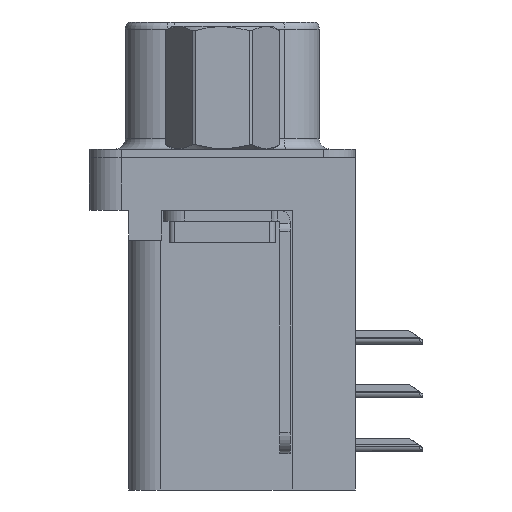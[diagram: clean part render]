
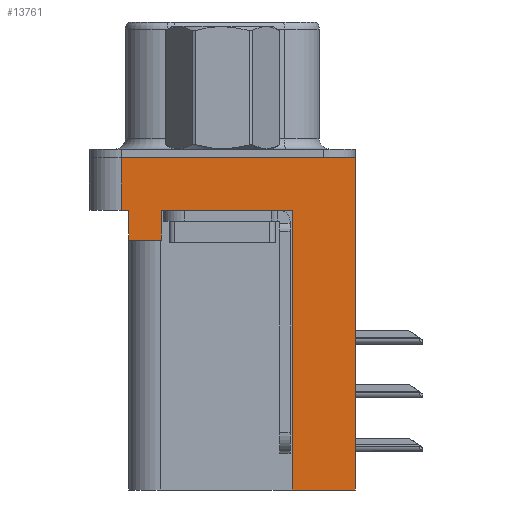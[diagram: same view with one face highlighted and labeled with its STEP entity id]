
A CAD part, left-side view. The second image highlights one B-rep face of the part: STEP entity #13761.
In plain terms, the highlighted planar face has unit normal (-1, 0, 0).
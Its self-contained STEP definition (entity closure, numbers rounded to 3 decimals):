
#424 = VERTEX_POINT ( 'NONE', #17950 ) ;
#439 = CARTESIAN_POINT ( 'NONE',  ( -2.91, 4.425, -3.9 ) ) ;
#512 = LINE ( 'NONE', #6853, #30821 ) ;
#1835 = EDGE_CURVE ( 'NONE', #17259, #18678, #512, .T. ) ;
#2288 = VECTOR ( 'NONE', #24441, 1000. ) ;
#3226 = CARTESIAN_POINT ( 'NONE',  ( -2.91, 4.425, -3.9 ) ) ;
#3287 = VERTEX_POINT ( 'NONE', #3580 ) ;
#3580 = CARTESIAN_POINT ( 'NONE',  ( -2.91, -3.295, -2.5 ) ) ;
#4330 = CARTESIAN_POINT ( 'NONE',  ( -2.91, -3.295, -15.7 ) ) ;
#4665 = ORIENTED_EDGE ( 'NONE', *, *, #38914, .T. ) ;
#4930 = CARTESIAN_POINT ( 'NONE',  ( -2.91, 4.775, -2.5 ) ) ;
#5229 = DIRECTION ( 'NONE',  ( 0., 0., 1. ) ) ;
#5302 = EDGE_CURVE ( 'NONE', #17259, #13470, #11109, .T. ) ;
#5963 = CARTESIAN_POINT ( 'NONE',  ( -2.91, 2.895, -2.5 ) ) ;
#6119 = ORIENTED_EDGE ( 'NONE', *, *, #8988, .F. ) ;
#6169 = DIRECTION ( 'NONE',  ( 0., 0., 1. ) ) ;
#6502 = DIRECTION ( 'NONE',  ( 0., 0., 1. ) ) ;
#6520 = CARTESIAN_POINT ( 'NONE',  ( -2.91, 4.775, 0. ) ) ;
#6759 = AXIS2_PLACEMENT_3D ( 'NONE', #12390, #24527, #6502 ) ;
#6853 = CARTESIAN_POINT ( 'NONE',  ( -2.91, 2.895, -3.9 ) ) ;
#7241 = EDGE_CURVE ( 'NONE', #424, #34237, #39481, .T. ) ;
#7870 = DIRECTION ( 'NONE',  ( 0., 0., 1. ) ) ;
#8988 = EDGE_CURVE ( 'NONE', #25546, #35656, #13294, .T. ) ;
#9423 = LINE ( 'NONE', #17387, #32931 ) ;
#9431 = ORIENTED_EDGE ( 'NONE', *, *, #9508, .F. ) ;
#9508 = EDGE_CURVE ( 'NONE', #424, #25546, #15098, .T. ) ;
#9706 = DIRECTION ( 'NONE',  ( 0., 0., 1. ) ) ;
#9744 = EDGE_CURVE ( 'NONE', #13470, #34237, #10437, .T. ) ;
#10287 = EDGE_CURVE ( 'NONE', #25316, #3287, #9423, .T. ) ;
#10437 = LINE ( 'NONE', #3226, #25574 ) ;
#10825 = EDGE_CURVE ( 'NONE', #34011, #25316, #37841, .T. ) ;
#11051 = EDGE_CURVE ( 'NONE', #34011, #35656, #38979, .T. ) ;
#11109 = LINE ( 'NONE', #439, #2288 ) ;
#11117 = ORIENTED_EDGE ( 'NONE', *, *, #5302, .F. ) ;
#11288 = ORIENTED_EDGE ( 'NONE', *, *, #11051, .T. ) ;
#12390 = CARTESIAN_POINT ( 'NONE',  ( -2.91, -6.275, -2.5 ) ) ;
#13294 = LINE ( 'NONE', #30433, #36029 ) ;
#13470 = VERTEX_POINT ( 'NONE', #31010 ) ;
#13516 = CARTESIAN_POINT ( 'NONE',  ( -2.91, 4.425, -2.5 ) ) ;
#13761 = ADVANCED_FACE ( 'NONE', ( #30510 ), #21433, .T. ) ;
#14116 = VECTOR ( 'NONE', #16298, 1000. ) ;
#15098 = LINE ( 'NONE', #4930, #30489 ) ;
#15733 = CARTESIAN_POINT ( 'NONE',  ( -2.91, -6.275, -2.5 ) ) ;
#16298 = DIRECTION ( 'NONE',  ( 0., 1., 0. ) ) ;
#16549 = LINE ( 'NONE', #24959, #23657 ) ;
#17077 = CARTESIAN_POINT ( 'NONE',  ( -2.91, -6.275, -2.5 ) ) ;
#17259 = VERTEX_POINT ( 'NONE', #36626 ) ;
#17279 = CARTESIAN_POINT ( 'NONE',  ( -2.91, -3.295, -15.7 ) ) ;
#17387 = CARTESIAN_POINT ( 'NONE',  ( -2.91, -3.295, -15.7 ) ) ;
#17950 = CARTESIAN_POINT ( 'NONE',  ( -2.91, 4.775, -2.5 ) ) ;
#18678 = VERTEX_POINT ( 'NONE', #5963 ) ;
#19077 = DIRECTION ( 'NONE',  ( 0., -1., 0. ) ) ;
#20397 = DIRECTION ( 'NONE',  ( 0., 0., 1. ) ) ;
#21433 = PLANE ( 'NONE',  #6759 ) ;
#23657 = VECTOR ( 'NONE', #19077, 1000. ) ;
#24296 = ORIENTED_EDGE ( 'NONE', *, *, #10825, .F. ) ;
#24441 = DIRECTION ( 'NONE',  ( 0., 1., 0. ) ) ;
#24527 = DIRECTION ( 'NONE',  ( -1., 0., 0. ) ) ;
#24959 = CARTESIAN_POINT ( 'NONE',  ( -2.91, -6.275, -2.5 ) ) ;
#25316 = VERTEX_POINT ( 'NONE', #17279 ) ;
#25546 = VERTEX_POINT ( 'NONE', #6520 ) ;
#25574 = VECTOR ( 'NONE', #6169, 1000. ) ;
#27241 = CARTESIAN_POINT ( 'NONE',  ( -2.91, -6.275, -15.7 ) ) ;
#28014 = ORIENTED_EDGE ( 'NONE', *, *, #1835, .T. ) ;
#30433 = CARTESIAN_POINT ( 'NONE',  ( -2.91, -6.275, 0. ) ) ;
#30489 = VECTOR ( 'NONE', #7870, 1000. ) ;
#30510 = FACE_OUTER_BOUND ( 'NONE', #39090, .T. ) ;
#30581 = VECTOR ( 'NONE', #5229, 1000. ) ;
#30821 = VECTOR ( 'NONE', #9706, 1000. ) ;
#31010 = CARTESIAN_POINT ( 'NONE',  ( -2.91, 4.425, -3.9 ) ) ;
#31056 = DIRECTION ( 'NONE',  ( 0., -1., 0. ) ) ;
#31685 = ORIENTED_EDGE ( 'NONE', *, *, #7241, .T. ) ;
#32931 = VECTOR ( 'NONE', #20397, 1000. ) ;
#33631 = DIRECTION ( 'NONE',  ( 0., -1., 0. ) ) ;
#34011 = VERTEX_POINT ( 'NONE', #27241 ) ;
#34237 = VERTEX_POINT ( 'NONE', #13516 ) ;
#35656 = VERTEX_POINT ( 'NONE', #36658 ) ;
#36029 = VECTOR ( 'NONE', #33631, 1000. ) ;
#36626 = CARTESIAN_POINT ( 'NONE',  ( -2.91, 2.895, -3.9 ) ) ;
#36658 = CARTESIAN_POINT ( 'NONE',  ( -2.91, -6.275, 0. ) ) ;
#37841 = LINE ( 'NONE', #4330, #14116 ) ;
#38540 = VECTOR ( 'NONE', #31056, 1000. ) ;
#38914 = EDGE_CURVE ( 'NONE', #18678, #3287, #16549, .T. ) ;
#38979 = LINE ( 'NONE', #17077, #30581 ) ;
#39090 = EDGE_LOOP ( 'NONE', ( #6119, #9431, #31685, #39370, #11117, #28014, #4665, #39147, #24296, #11288 ) ) ;
#39147 = ORIENTED_EDGE ( 'NONE', *, *, #10287, .F. ) ;
#39370 = ORIENTED_EDGE ( 'NONE', *, *, #9744, .F. ) ;
#39481 = LINE ( 'NONE', #15733, #38540 ) ;
